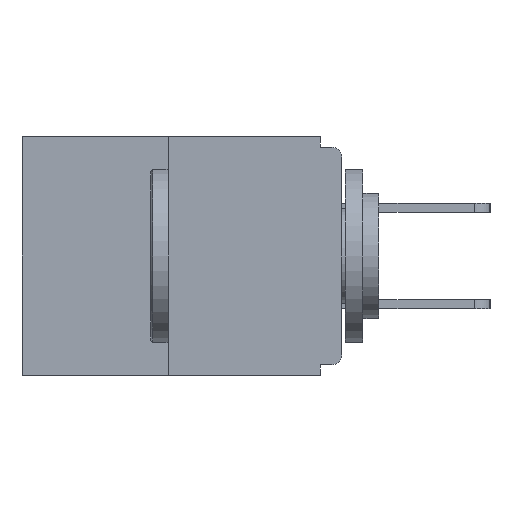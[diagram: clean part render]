
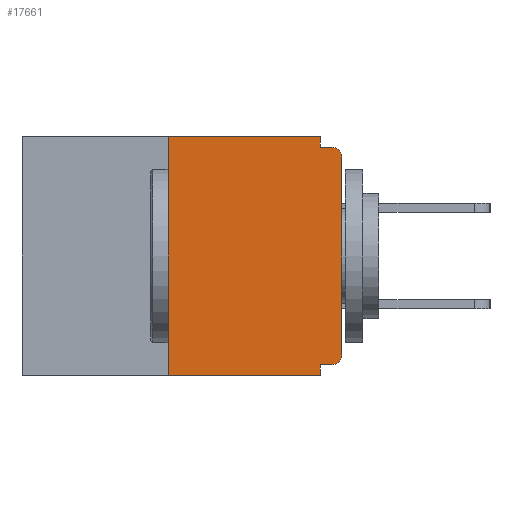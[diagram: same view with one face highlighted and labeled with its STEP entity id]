
A CAD part, left-side view. The second image highlights one B-rep face of the part: STEP entity #17661.
In plain terms, the highlighted planar face has unit normal (-1, 0, 0).
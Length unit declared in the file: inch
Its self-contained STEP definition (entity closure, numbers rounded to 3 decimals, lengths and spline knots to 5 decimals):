
#482 = VERTEX_POINT ( 'NONE', #21232 ) ;
#680 = EDGE_CURVE ( 'NONE', #16991, #3036, #12029, .T. ) ;
#1121 = VERTEX_POINT ( 'NONE', #15112 ) ;
#1777 = DIRECTION ( 'NONE',  ( 0., 0., 1. ) ) ;
#2233 = LINE ( 'NONE', #13486, #4054 ) ;
#2513 = LINE ( 'NONE', #9287, #15135 ) ;
#3036 = VERTEX_POINT ( 'NONE', #20499 ) ;
#3046 = ORIENTED_EDGE ( 'NONE', *, *, #7571, .F. ) ;
#3093 = CARTESIAN_POINT ( 'NONE',  ( 0., 0.015, -0.015 ) ) ;
#3445 = CARTESIAN_POINT ( 'NONE',  ( 0., 0.015, -0.03 ) ) ;
#3980 = PLANE ( 'NONE',  #8970 ) ;
#4015 = ORIENTED_EDGE ( 'NONE', *, *, #5348, .T. ) ;
#4054 = VECTOR ( 'NONE', #1777, 39.37008 ) ;
#4456 = CIRCLE ( 'NONE', #8397, 0.015 ) ;
#4511 = DIRECTION ( 'NONE',  ( 0., -1., 0. ) ) ;
#4544 = VECTOR ( 'NONE', #7086, 39.37008 ) ;
#5067 = DIRECTION ( 'NONE',  ( 0., 0., -1. ) ) ;
#5143 = CARTESIAN_POINT ( 'NONE',  ( 0., 0.031, 0. ) ) ;
#5348 = EDGE_CURVE ( 'NONE', #12292, #19647, #4456, .T. ) ;
#5382 = CARTESIAN_POINT ( 'NONE',  ( 0., 0.015, -0.328 ) ) ;
#5391 = AXIS2_PLACEMENT_3D ( 'NONE', #15209, #6879, #11721 ) ;
#5642 = ORIENTED_EDGE ( 'NONE', *, *, #17022, .F. ) ;
#5652 = DIRECTION ( 'NONE',  ( 0., 0., -1. ) ) ;
#6029 = DIRECTION ( 'NONE',  ( 0., 0., -1. ) ) ;
#6164 = DIRECTION ( 'NONE',  ( 0., -1., 0. ) ) ;
#6537 = EDGE_CURVE ( 'NONE', #14767, #19367, #13905, .T. ) ;
#6879 = DIRECTION ( 'NONE',  ( -1., 0., 0. ) ) ;
#7086 = DIRECTION ( 'NONE',  ( 0., 0., 1. ) ) ;
#7315 = ORIENTED_EDGE ( 'NONE', *, *, #10209, .F. ) ;
#7571 = EDGE_CURVE ( 'NONE', #16298, #9496, #2513, .T. ) ;
#7843 = VECTOR ( 'NONE', #20636, 39.37008 ) ;
#8397 = AXIS2_PLACEMENT_3D ( 'NONE', #3445, #18338, #5067 ) ;
#8779 = DIRECTION ( 'NONE',  ( 0., 1., 0. ) ) ;
#8884 = DIRECTION ( 'NONE',  ( 1., 0., 0. ) ) ;
#8962 = CARTESIAN_POINT ( 'NONE',  ( 0., 0.46, 0. ) ) ;
#8970 = AXIS2_PLACEMENT_3D ( 'NONE', #8962, #8884, #5652 ) ;
#9287 = CARTESIAN_POINT ( 'NONE',  ( 0., 0.031, -0.343 ) ) ;
#9496 = VERTEX_POINT ( 'NONE', #11819 ) ;
#9505 = CARTESIAN_POINT ( 'NONE',  ( 0., 0.46, 0. ) ) ;
#10113 = EDGE_CURVE ( 'NONE', #19367, #12292, #20030, .T. ) ;
#10193 = CARTESIAN_POINT ( 'NONE',  ( 0., 0., -0.03 ) ) ;
#10209 = EDGE_CURVE ( 'NONE', #3036, #19647, #15591, .T. ) ;
#10232 = LINE ( 'NONE', #9505, #16894 ) ;
#10304 = VECTOR ( 'NONE', #8779, 39.37008 ) ;
#10487 = VECTOR ( 'NONE', #4511, 39.37008 ) ;
#10516 = CARTESIAN_POINT ( 'NONE',  ( 0., 0., 0. ) ) ;
#10677 = CARTESIAN_POINT ( 'NONE',  ( 0., 0.031, 0. ) ) ;
#10798 = ORIENTED_EDGE ( 'NONE', *, *, #16218, .F. ) ;
#10955 = ORIENTED_EDGE ( 'NONE', *, *, #10113, .T. ) ;
#11125 = ORIENTED_EDGE ( 'NONE', *, *, #11732, .T. ) ;
#11721 = DIRECTION ( 'NONE',  ( 0., 0., -1. ) ) ;
#11732 = EDGE_CURVE ( 'NONE', #482, #9496, #20470, .T. ) ;
#11819 = CARTESIAN_POINT ( 'NONE',  ( 0., 0.031, -0.343 ) ) ;
#11962 = VECTOR ( 'NONE', #12135, 39.37008 ) ;
#12029 = LINE ( 'NONE', #5143, #7843 ) ;
#12135 = DIRECTION ( 'NONE',  ( 0., -1., 0. ) ) ;
#12292 = VERTEX_POINT ( 'NONE', #10193 ) ;
#13165 = EDGE_LOOP ( 'NONE', ( #5642, #15563, #11125, #3046, #10798, #17714, #10955, #4015, #7315, #14399 ) ) ;
#13486 = CARTESIAN_POINT ( 'NONE',  ( 0., 0.25, 0. ) ) ;
#13621 = CARTESIAN_POINT ( 'NONE',  ( 0., 0., -0.328 ) ) ;
#13905 = CIRCLE ( 'NONE', #5391, 0.015 ) ;
#14399 = ORIENTED_EDGE ( 'NONE', *, *, #680, .F. ) ;
#14767 = VERTEX_POINT ( 'NONE', #5382 ) ;
#15112 = CARTESIAN_POINT ( 'NONE',  ( 0., 0.25, 0. ) ) ;
#15135 = VECTOR ( 'NONE', #6029, 39.37008 ) ;
#15209 = CARTESIAN_POINT ( 'NONE',  ( 0., 0.015, -0.313 ) ) ;
#15336 = CARTESIAN_POINT ( 'NONE',  ( 0., 0.46, -0.343 ) ) ;
#15563 = ORIENTED_EDGE ( 'NONE', *, *, #16040, .F. ) ;
#15591 = LINE ( 'NONE', #19236, #10487 ) ;
#16040 = EDGE_CURVE ( 'NONE', #482, #1121, #2233, .T. ) ;
#16218 = EDGE_CURVE ( 'NONE', #14767, #16298, #19059, .T. ) ;
#16298 = VERTEX_POINT ( 'NONE', #20484 ) ;
#16894 = VECTOR ( 'NONE', #6164, 39.37008 ) ;
#16991 = VERTEX_POINT ( 'NONE', #10677 ) ;
#17022 = EDGE_CURVE ( 'NONE', #1121, #16991, #10232, .T. ) ;
#17661 = ADVANCED_FACE ( 'NONE', ( #20556 ), #3980, .F. ) ;
#17714 = ORIENTED_EDGE ( 'NONE', *, *, #6537, .T. ) ;
#18338 = DIRECTION ( 'NONE',  ( -1., 0., 0. ) ) ;
#19059 = LINE ( 'NONE', #13621, #10304 ) ;
#19236 = CARTESIAN_POINT ( 'NONE',  ( 0., 0., -0.015 ) ) ;
#19367 = VERTEX_POINT ( 'NONE', #20514 ) ;
#19647 = VERTEX_POINT ( 'NONE', #3093 ) ;
#20030 = LINE ( 'NONE', #10516, #4544 ) ;
#20470 = LINE ( 'NONE', #15336, #11962 ) ;
#20484 = CARTESIAN_POINT ( 'NONE',  ( 0., 0.031, -0.328 ) ) ;
#20499 = CARTESIAN_POINT ( 'NONE',  ( 0., 0.031, -0.015 ) ) ;
#20514 = CARTESIAN_POINT ( 'NONE',  ( 0., 0., -0.313 ) ) ;
#20556 = FACE_OUTER_BOUND ( 'NONE', #13165, .T. ) ;
#20636 = DIRECTION ( 'NONE',  ( 0., 0., -1. ) ) ;
#21232 = CARTESIAN_POINT ( 'NONE',  ( 0., 0.25, -0.343 ) ) ;
